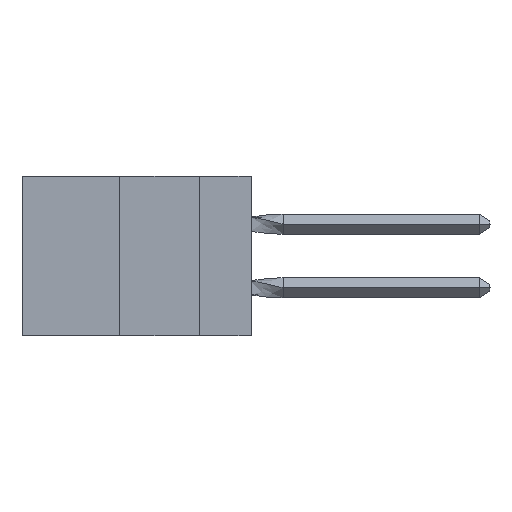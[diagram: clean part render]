
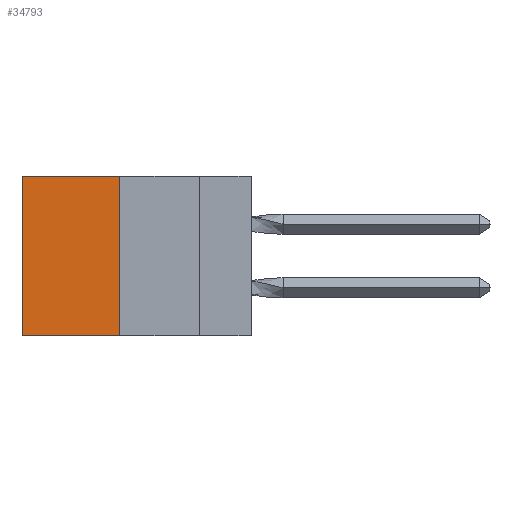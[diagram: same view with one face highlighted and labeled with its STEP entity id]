
A CAD part, left-side view. The second image highlights one B-rep face of the part: STEP entity #34793.
In plain terms, the highlighted planar face has unit normal (-1, 0, 0).
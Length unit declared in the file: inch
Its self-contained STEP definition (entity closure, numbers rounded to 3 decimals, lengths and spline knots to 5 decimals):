
#218 = PLANE ( 'NONE',  #37473 ) ;
#353 = CARTESIAN_POINT ( 'NONE',  ( 0.305, 0.413, -0.5 ) ) ;
#1918 = DIRECTION ( 'NONE',  ( 0., 0., -1. ) ) ;
#2836 = LINE ( 'NONE', #24855, #14086 ) ;
#3494 = VECTOR ( 'NONE', #1918, 39.37008 ) ;
#3894 = EDGE_CURVE ( 'NONE', #6551, #7707, #20047, .T. ) ;
#3996 = ORIENTED_EDGE ( 'NONE', *, *, #12463, .F. ) ;
#4846 = VECTOR ( 'NONE', #25175, 39.37008 ) ;
#5544 = ORIENTED_EDGE ( 'NONE', *, *, #16488, .F. ) ;
#6551 = VERTEX_POINT ( 'NONE', #20943 ) ;
#7065 = ORIENTED_EDGE ( 'NONE', *, *, #3894, .T. ) ;
#7707 = VERTEX_POINT ( 'NONE', #33574 ) ;
#8382 = ORIENTED_EDGE ( 'NONE', *, *, #14397, .T. ) ;
#8981 = DIRECTION ( 'NONE',  ( 1., 0., 0. ) ) ;
#9006 = LINE ( 'NONE', #36748, #4846 ) ;
#12463 = EDGE_CURVE ( 'NONE', #31820, #14712, #9006, .T. ) ;
#13928 = CARTESIAN_POINT ( 'NONE',  ( 0.305, 0.413, 0. ) ) ;
#14086 = VECTOR ( 'NONE', #28172, 39.37008 ) ;
#14397 = EDGE_CURVE ( 'NONE', #7707, #14712, #2836, .T. ) ;
#14712 = VERTEX_POINT ( 'NONE', #25229 ) ;
#15698 = FACE_OUTER_BOUND ( 'NONE', #31478, .T. ) ;
#16488 = EDGE_CURVE ( 'NONE', #6551, #31820, #27898, .T. ) ;
#16745 = CARTESIAN_POINT ( 'NONE',  ( 0.305, 0.413, -0.5 ) ) ;
#20047 = LINE ( 'NONE', #13928, #38795 ) ;
#20943 = CARTESIAN_POINT ( 'NONE',  ( 0.305, 0.413, 0. ) ) ;
#21310 = DIRECTION ( 'NONE',  ( 0., 0., -1. ) ) ;
#24855 = CARTESIAN_POINT ( 'NONE',  ( 0.305, 0.72, -0.5 ) ) ;
#25175 = DIRECTION ( 'NONE',  ( 0., 1., 0. ) ) ;
#25229 = CARTESIAN_POINT ( 'NONE',  ( 0.305, 0.72, -0.5 ) ) ;
#27898 = LINE ( 'NONE', #28779, #3494 ) ;
#28172 = DIRECTION ( 'NONE',  ( 0., 0., -1. ) ) ;
#28779 = CARTESIAN_POINT ( 'NONE',  ( 0.305, 0.413, -0.5 ) ) ;
#31478 = EDGE_LOOP ( 'NONE', ( #8382, #3996, #5544, #7065 ) ) ;
#31820 = VERTEX_POINT ( 'NONE', #16745 ) ;
#33574 = CARTESIAN_POINT ( 'NONE',  ( 0.305, 0.72, 0. ) ) ;
#34793 = ADVANCED_FACE ( 'NONE', ( #15698 ), #218, .F. ) ;
#34923 = DIRECTION ( 'NONE',  ( 0., 1., 0. ) ) ;
#36748 = CARTESIAN_POINT ( 'NONE',  ( 0.305, 0.413, -0.5 ) ) ;
#37473 = AXIS2_PLACEMENT_3D ( 'NONE', #353, #8981, #21310 ) ;
#38795 = VECTOR ( 'NONE', #34923, 39.37008 ) ;
